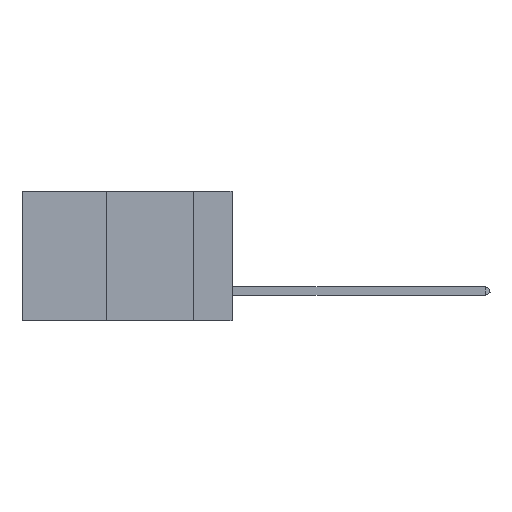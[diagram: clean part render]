
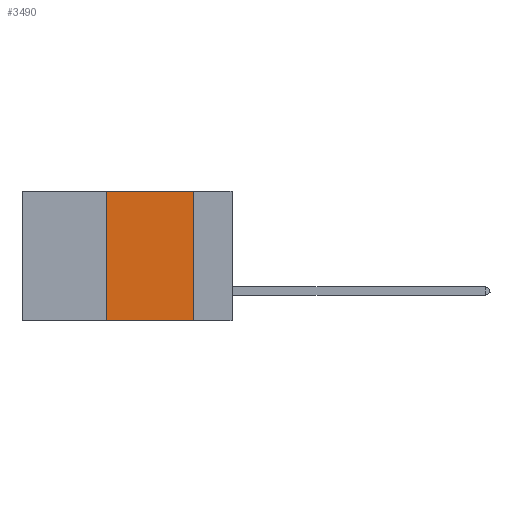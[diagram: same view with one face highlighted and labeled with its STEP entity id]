
A CAD part, left-side view. The second image highlights one B-rep face of the part: STEP entity #3490.
In plain terms, the highlighted planar face has unit normal (-1, 0, 0).
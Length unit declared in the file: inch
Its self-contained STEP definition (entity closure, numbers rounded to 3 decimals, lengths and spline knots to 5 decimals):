
#349 = LINE ( 'NONE', #25425, #11187 ) ;
#1388 = ORIENTED_EDGE ( 'NONE', *, *, #1853, .F. ) ;
#1853 = EDGE_CURVE ( 'NONE', #4349, #6395, #11863, .T. ) ;
#2358 = FACE_OUTER_BOUND ( 'NONE', #14430, .T. ) ;
#2377 = PLANE ( 'NONE',  #21828 ) ;
#2458 = CARTESIAN_POINT ( 'NONE',  ( 0., 0.6, 0. ) ) ;
#2711 = CARTESIAN_POINT ( 'NONE',  ( 0., 0.11, -0.37 ) ) ;
#2717 = LINE ( 'NONE', #21967, #8171 ) ;
#3490 = ADVANCED_FACE ( 'NONE', ( #2358 ), #2377, .F. ) ;
#4349 = VERTEX_POINT ( 'NONE', #5920 ) ;
#5004 = VECTOR ( 'NONE', #29839, 39.37008 ) ;
#5327 = ORIENTED_EDGE ( 'NONE', *, *, #26765, .T. ) ;
#5920 = CARTESIAN_POINT ( 'NONE',  ( 0., 0.36, 0. ) ) ;
#6395 = VERTEX_POINT ( 'NONE', #18458 ) ;
#7133 = DIRECTION ( 'NONE',  ( 1., 0., 0. ) ) ;
#8171 = VECTOR ( 'NONE', #24528, 39.37008 ) ;
#9778 = DIRECTION ( 'NONE',  ( 0., -1., 0. ) ) ;
#10891 = EDGE_CURVE ( 'NONE', #12043, #4349, #2717, .T. ) ;
#10973 = LINE ( 'NONE', #19344, #23236 ) ;
#11175 = ORIENTED_EDGE ( 'NONE', *, *, #21880, .F. ) ;
#11187 = VECTOR ( 'NONE', #11829, 39.37008 ) ;
#11298 = CARTESIAN_POINT ( 'NONE',  ( 0., 0.6, 0. ) ) ;
#11829 = DIRECTION ( 'NONE',  ( 0., 0., -1. ) ) ;
#11863 = LINE ( 'NONE', #11298, #5004 ) ;
#12043 = VERTEX_POINT ( 'NONE', #21231 ) ;
#14430 = EDGE_LOOP ( 'NONE', ( #11175, #1388, #21757, #5327 ) ) ;
#18458 = CARTESIAN_POINT ( 'NONE',  ( 0., 0.11, 0. ) ) ;
#19344 = CARTESIAN_POINT ( 'NONE',  ( 0., 0.6, -0.37 ) ) ;
#21231 = CARTESIAN_POINT ( 'NONE',  ( 0., 0.36, -0.37 ) ) ;
#21757 = ORIENTED_EDGE ( 'NONE', *, *, #10891, .F. ) ;
#21828 = AXIS2_PLACEMENT_3D ( 'NONE', #2458, #7133, #27887 ) ;
#21880 = EDGE_CURVE ( 'NONE', #6395, #28306, #349, .T. ) ;
#21967 = CARTESIAN_POINT ( 'NONE',  ( 0., 0.36, 0. ) ) ;
#23236 = VECTOR ( 'NONE', #9778, 39.37008 ) ;
#24528 = DIRECTION ( 'NONE',  ( 0., 0., 1. ) ) ;
#25425 = CARTESIAN_POINT ( 'NONE',  ( 0., 0.11, 0. ) ) ;
#26765 = EDGE_CURVE ( 'NONE', #12043, #28306, #10973, .T. ) ;
#27887 = DIRECTION ( 'NONE',  ( 0., 0., -1. ) ) ;
#28306 = VERTEX_POINT ( 'NONE', #2711 ) ;
#29839 = DIRECTION ( 'NONE',  ( 0., -1., 0. ) ) ;
